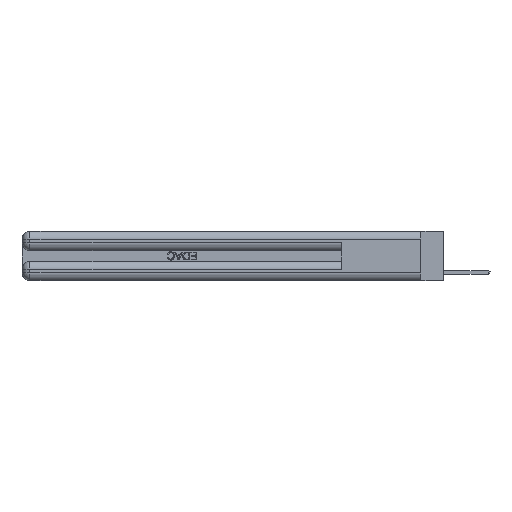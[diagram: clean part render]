
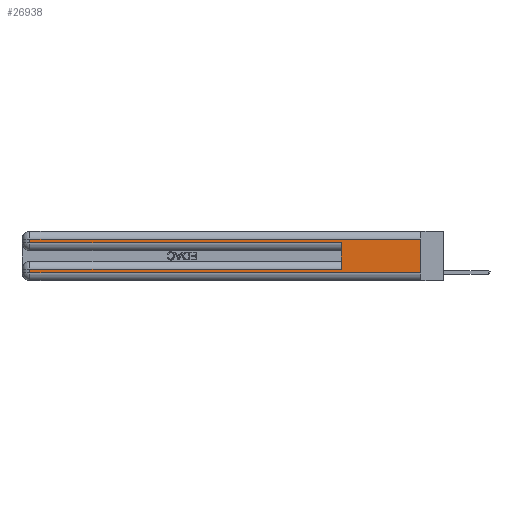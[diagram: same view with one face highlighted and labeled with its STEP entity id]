
A CAD part, left-side view. The second image highlights one B-rep face of the part: STEP entity #26938.
In plain terms, the highlighted planar face has unit normal (-1, 0, 0).
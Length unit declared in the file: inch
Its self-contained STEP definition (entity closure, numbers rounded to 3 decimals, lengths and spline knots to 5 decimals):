
#161 = EDGE_CURVE ( 'NONE', #17225, #6085, #19024, .T. ) ;
#203 = EDGE_CURVE ( 'NONE', #17225, #12550, #927, .T. ) ;
#357 = ORIENTED_EDGE ( 'NONE', *, *, #161, .T. ) ;
#558 = VECTOR ( 'NONE', #10087, 39.37008 ) ;
#714 = CARTESIAN_POINT ( 'NONE',  ( 0., 0., 0.31 ) ) ;
#927 = LINE ( 'NONE', #18022, #2338 ) ;
#980 = VECTOR ( 'NONE', #21694, 39.37008 ) ;
#1130 = DIRECTION ( 'NONE',  ( 0., -1., 0. ) ) ;
#1661 = LINE ( 'NONE', #16374, #558 ) ;
#1863 = CARTESIAN_POINT ( 'NONE',  ( 0., 0., 0.37 ) ) ;
#2338 = VECTOR ( 'NONE', #15507, 39.37008 ) ;
#3183 = VECTOR ( 'NONE', #4593, 39.37008 ) ;
#3254 = ORIENTED_EDGE ( 'NONE', *, *, #17889, .F. ) ;
#4267 = VERTEX_POINT ( 'NONE', #8283 ) ;
#4593 = DIRECTION ( 'NONE',  ( 0., 0., -1. ) ) ;
#5156 = CARTESIAN_POINT ( 'NONE',  ( 0., 0., 0.285 ) ) ;
#6085 = VERTEX_POINT ( 'NONE', #23228 ) ;
#6470 = CARTESIAN_POINT ( 'NONE',  ( 0., 2.94, 0.285 ) ) ;
#6921 = LINE ( 'NONE', #714, #980 ) ;
#6952 = EDGE_CURVE ( 'NONE', #4267, #14414, #22325, .T. ) ;
#7705 = DIRECTION ( 'NONE',  ( 0., -1., 0. ) ) ;
#8283 = CARTESIAN_POINT ( 'NONE',  ( 0., 2.94, 0.31 ) ) ;
#8351 = DIRECTION ( 'NONE',  ( 1., 0., 0. ) ) ;
#8704 = ORIENTED_EDGE ( 'NONE', *, *, #23068, .T. ) ;
#8750 = CARTESIAN_POINT ( 'NONE',  ( 0., 0., 0.31 ) ) ;
#8950 = VECTOR ( 'NONE', #26763, 39.37008 ) ;
#9006 = LINE ( 'NONE', #5156, #19975 ) ;
#9120 = LINE ( 'NONE', #23377, #3183 ) ;
#10087 = DIRECTION ( 'NONE',  ( 0., 0., -1. ) ) ;
#11720 = CARTESIAN_POINT ( 'NONE',  ( 0., 2.94, 0.37 ) ) ;
#11852 = CARTESIAN_POINT ( 'NONE',  ( 0., 0.6, 0.285 ) ) ;
#12550 = VERTEX_POINT ( 'NONE', #11852 ) ;
#12806 = CARTESIAN_POINT ( 'NONE',  ( 0., 0.6, 0.085 ) ) ;
#12934 = DIRECTION ( 'NONE',  ( 0., 0., -1. ) ) ;
#13974 = CARTESIAN_POINT ( 'NONE',  ( 0., 0., 0.06 ) ) ;
#14414 = VERTEX_POINT ( 'NONE', #6470 ) ;
#14489 = ORIENTED_EDGE ( 'NONE', *, *, #17670, .T. ) ;
#14613 = EDGE_LOOP ( 'NONE', ( #3254, #14489, #25477, #18639, #20322, #357, #8704, #15903 ) ) ;
#15435 = CARTESIAN_POINT ( 'NONE',  ( 0., 0., 0.06 ) ) ;
#15507 = DIRECTION ( 'NONE',  ( 0., 0., 1. ) ) ;
#15903 = ORIENTED_EDGE ( 'NONE', *, *, #21555, .T. ) ;
#16374 = CARTESIAN_POINT ( 'NONE',  ( 0., 0., 0.37 ) ) ;
#16590 = PLANE ( 'NONE',  #22938 ) ;
#16976 = VECTOR ( 'NONE', #21251, 39.37008 ) ;
#17225 = VERTEX_POINT ( 'NONE', #12806 ) ;
#17670 = EDGE_CURVE ( 'NONE', #24758, #4267, #6921, .T. ) ;
#17889 = EDGE_CURVE ( 'NONE', #24758, #21351, #1661, .T. ) ;
#18022 = CARTESIAN_POINT ( 'NONE',  ( 0., 0.6, 0.145 ) ) ;
#18167 = LINE ( 'NONE', #13974, #25410 ) ;
#18639 = ORIENTED_EDGE ( 'NONE', *, *, #19859, .T. ) ;
#18971 = FACE_OUTER_BOUND ( 'NONE', #14613, .T. ) ;
#19024 = LINE ( 'NONE', #21661, #16976 ) ;
#19176 = CARTESIAN_POINT ( 'NONE',  ( 0., 2.94, 0.06 ) ) ;
#19859 = EDGE_CURVE ( 'NONE', #14414, #12550, #9006, .T. ) ;
#19975 = VECTOR ( 'NONE', #1130, 39.37008 ) ;
#20132 = VERTEX_POINT ( 'NONE', #19176 ) ;
#20322 = ORIENTED_EDGE ( 'NONE', *, *, #203, .F. ) ;
#21251 = DIRECTION ( 'NONE',  ( 0., 1., 0. ) ) ;
#21351 = VERTEX_POINT ( 'NONE', #15435 ) ;
#21555 = EDGE_CURVE ( 'NONE', #20132, #21351, #18167, .T. ) ;
#21661 = CARTESIAN_POINT ( 'NONE',  ( 0., 0., 0.085 ) ) ;
#21694 = DIRECTION ( 'NONE',  ( 0., 1., 0. ) ) ;
#22325 = LINE ( 'NONE', #11720, #8950 ) ;
#22938 = AXIS2_PLACEMENT_3D ( 'NONE', #1863, #8351, #12934 ) ;
#23068 = EDGE_CURVE ( 'NONE', #6085, #20132, #9120, .T. ) ;
#23228 = CARTESIAN_POINT ( 'NONE',  ( 0., 2.94, 0.085 ) ) ;
#23377 = CARTESIAN_POINT ( 'NONE',  ( 0., 2.94, 0.37 ) ) ;
#24758 = VERTEX_POINT ( 'NONE', #8750 ) ;
#25410 = VECTOR ( 'NONE', #7705, 39.37008 ) ;
#25477 = ORIENTED_EDGE ( 'NONE', *, *, #6952, .T. ) ;
#26763 = DIRECTION ( 'NONE',  ( 0., 0., -1. ) ) ;
#26938 = ADVANCED_FACE ( 'NONE', ( #18971 ), #16590, .F. ) ;
